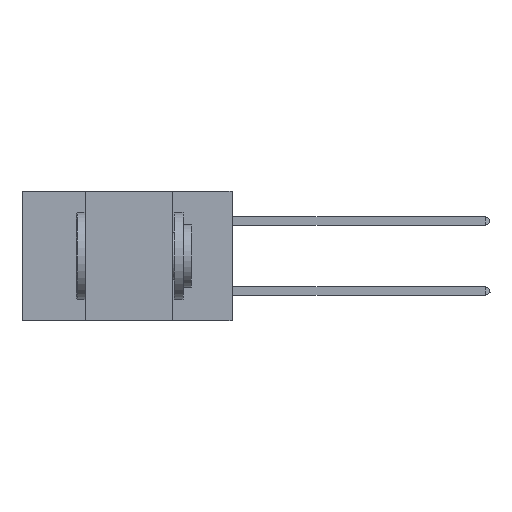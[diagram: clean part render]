
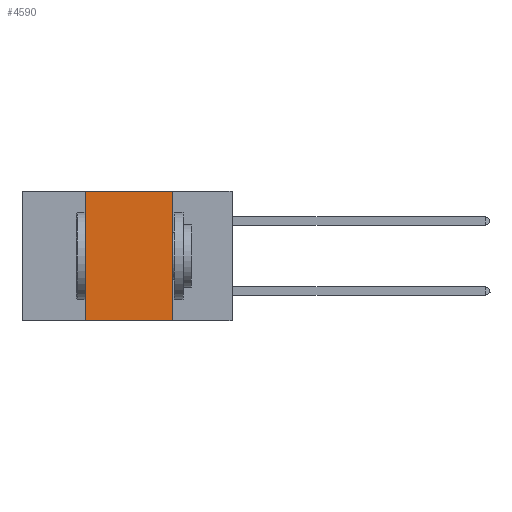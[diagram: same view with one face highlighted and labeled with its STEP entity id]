
A CAD part, left-side view. The second image highlights one B-rep face of the part: STEP entity #4590.
In plain terms, the highlighted planar face has unit normal (-1, 0, 0).
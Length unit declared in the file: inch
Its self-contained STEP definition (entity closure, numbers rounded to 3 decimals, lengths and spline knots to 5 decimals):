
#81 = LINE ( 'NONE', #16999, #4653 ) ;
#796 = LINE ( 'NONE', #3273, #16680 ) ;
#1133 = ORIENTED_EDGE ( 'NONE', *, *, #16234, .F. ) ;
#1265 = PLANE ( 'NONE',  #16777 ) ;
#1655 = EDGE_LOOP ( 'NONE', ( #4459, #1133, #18766, #14514 ) ) ;
#1802 = CARTESIAN_POINT ( 'NONE',  ( 0., 0.17, 0. ) ) ;
#2877 = CARTESIAN_POINT ( 'NONE',  ( 0., 0.6, 0. ) ) ;
#3273 = CARTESIAN_POINT ( 'NONE',  ( 0., 0.6, -0.37 ) ) ;
#3650 = VERTEX_POINT ( 'NONE', #6899 ) ;
#3761 = VERTEX_POINT ( 'NONE', #1802 ) ;
#4459 = ORIENTED_EDGE ( 'NONE', *, *, #6496, .F. ) ;
#4590 = ADVANCED_FACE ( 'NONE', ( #16257 ), #1265, .F. ) ;
#4653 = VECTOR ( 'NONE', #16855, 39.37008 ) ;
#6440 = CARTESIAN_POINT ( 'NONE',  ( 0., 0.42, 0. ) ) ;
#6496 = EDGE_CURVE ( 'NONE', #3761, #3650, #81, .T. ) ;
#6610 = VERTEX_POINT ( 'NONE', #12875 ) ;
#6899 = CARTESIAN_POINT ( 'NONE',  ( 0., 0.17, -0.37 ) ) ;
#6943 = DIRECTION ( 'NONE',  ( 0., 0., -1. ) ) ;
#7543 = LINE ( 'NONE', #6440, #8888 ) ;
#7916 = EDGE_CURVE ( 'NONE', #12025, #6610, #7543, .T. ) ;
#8420 = EDGE_CURVE ( 'NONE', #12025, #3650, #796, .T. ) ;
#8718 = LINE ( 'NONE', #2877, #12564 ) ;
#8888 = VECTOR ( 'NONE', #12260, 39.37008 ) ;
#10182 = DIRECTION ( 'NONE',  ( 0., -1., 0. ) ) ;
#12025 = VERTEX_POINT ( 'NONE', #18655 ) ;
#12260 = DIRECTION ( 'NONE',  ( 0., 0., 1. ) ) ;
#12564 = VECTOR ( 'NONE', #10182, 39.37008 ) ;
#12875 = CARTESIAN_POINT ( 'NONE',  ( 0., 0.42, 0. ) ) ;
#13344 = DIRECTION ( 'NONE',  ( 0., -1., 0. ) ) ;
#14514 = ORIENTED_EDGE ( 'NONE', *, *, #8420, .T. ) ;
#15773 = CARTESIAN_POINT ( 'NONE',  ( 0., 0.6, 0. ) ) ;
#16234 = EDGE_CURVE ( 'NONE', #6610, #3761, #8718, .T. ) ;
#16257 = FACE_OUTER_BOUND ( 'NONE', #1655, .T. ) ;
#16680 = VECTOR ( 'NONE', #13344, 39.37008 ) ;
#16777 = AXIS2_PLACEMENT_3D ( 'NONE', #15773, #17264, #6943 ) ;
#16855 = DIRECTION ( 'NONE',  ( 0., 0., -1. ) ) ;
#16999 = CARTESIAN_POINT ( 'NONE',  ( 0., 0.17, 0. ) ) ;
#17264 = DIRECTION ( 'NONE',  ( 1., 0., 0. ) ) ;
#18655 = CARTESIAN_POINT ( 'NONE',  ( 0., 0.42, -0.37 ) ) ;
#18766 = ORIENTED_EDGE ( 'NONE', *, *, #7916, .F. ) ;
